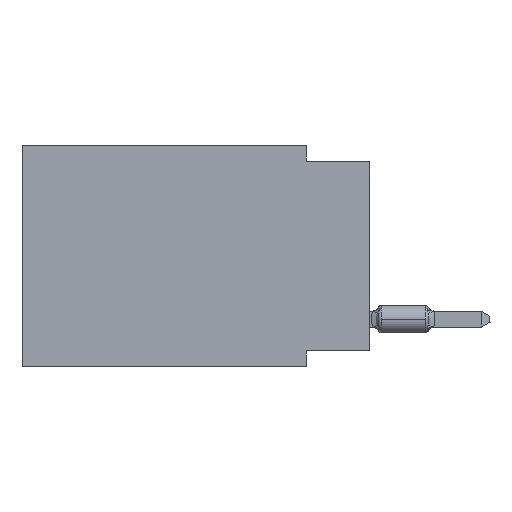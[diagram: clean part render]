
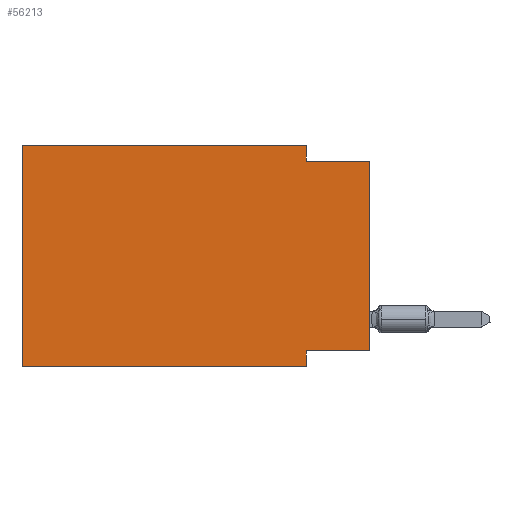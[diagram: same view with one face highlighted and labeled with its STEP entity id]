
A CAD part, left-side view. The second image highlights one B-rep face of the part: STEP entity #56213.
In plain terms, the highlighted planar face has unit normal (-1, 0, 0).
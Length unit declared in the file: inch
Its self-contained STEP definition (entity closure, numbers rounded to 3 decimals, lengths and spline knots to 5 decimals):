
#253 = VECTOR ( 'NONE', #26847, 39.37008 ) ;
#733 = VECTOR ( 'NONE', #78501, 39.37008 ) ;
#910 = LINE ( 'NONE', #87349, #33167 ) ;
#974 = VERTEX_POINT ( 'NONE', #85947 ) ;
#3097 = EDGE_LOOP ( 'NONE', ( #95310, #85120, #35525, #90242, #63247, #29142, #25572, #78518 ) ) ;
#9941 = DIRECTION ( 'NONE',  ( 0., 0., -1. ) ) ;
#10083 = CARTESIAN_POINT ( 'NONE',  ( 0., 0.1, 0. ) ) ;
#11758 = CARTESIAN_POINT ( 'NONE',  ( 0., 0.55, 0. ) ) ;
#11990 = EDGE_CURVE ( 'NONE', #82750, #92309, #94597, .T. ) ;
#13681 = VERTEX_POINT ( 'NONE', #62762 ) ;
#15347 = CARTESIAN_POINT ( 'NONE',  ( 0., 0.55, 0. ) ) ;
#17372 = DIRECTION ( 'NONE',  ( 0., 0., 1. ) ) ;
#17712 = EDGE_CURVE ( 'NONE', #47545, #46386, #76178, .T. ) ;
#20747 = DIRECTION ( 'NONE',  ( 0., -1., 0. ) ) ;
#23045 = EDGE_CURVE ( 'NONE', #47545, #87783, #51930, .T. ) ;
#25572 = ORIENTED_EDGE ( 'NONE', *, *, #84690, .F. ) ;
#26516 = CARTESIAN_POINT ( 'NONE',  ( 0., 0.55, -0.35 ) ) ;
#26847 = DIRECTION ( 'NONE',  ( 0., 1., 0. ) ) ;
#29142 = ORIENTED_EDGE ( 'NONE', *, *, #23045, .T. ) ;
#29228 = LINE ( 'NONE', #63686, #35225 ) ;
#31982 = VECTOR ( 'NONE', #103649, 39.37008 ) ;
#32868 = LINE ( 'NONE', #15347, #35991 ) ;
#33167 = VECTOR ( 'NONE', #9941, 39.37008 ) ;
#35225 = VECTOR ( 'NONE', #20747, 39.37008 ) ;
#35525 = ORIENTED_EDGE ( 'NONE', *, *, #102534, .F. ) ;
#35991 = VECTOR ( 'NONE', #67318, 39.37008 ) ;
#41147 = LINE ( 'NONE', #58653, #95939 ) ;
#46386 = VERTEX_POINT ( 'NONE', #98865 ) ;
#47545 = VERTEX_POINT ( 'NONE', #80386 ) ;
#50631 = LINE ( 'NONE', #85115, #253 ) ;
#51930 = LINE ( 'NONE', #26516, #733 ) ;
#54200 = VECTOR ( 'NONE', #17372, 39.37008 ) ;
#56213 = ADVANCED_FACE ( 'NONE', ( #89169 ), #103924, .F. ) ;
#58653 = CARTESIAN_POINT ( 'NONE',  ( 0., 0.1, 0. ) ) ;
#59770 = AXIS2_PLACEMENT_3D ( 'NONE', #11758, #69436, #60941 ) ;
#60941 = DIRECTION ( 'NONE',  ( 0., 0., -1. ) ) ;
#62762 = CARTESIAN_POINT ( 'NONE',  ( 0., 0.1, -0.025 ) ) ;
#63247 = ORIENTED_EDGE ( 'NONE', *, *, #17712, .F. ) ;
#63686 = CARTESIAN_POINT ( 'NONE',  ( 0., 0., -0.025 ) ) ;
#65373 = VERTEX_POINT ( 'NONE', #10083 ) ;
#67318 = DIRECTION ( 'NONE',  ( 0., -1., 0. ) ) ;
#69151 = CARTESIAN_POINT ( 'NONE',  ( 0., 0., 0. ) ) ;
#69436 = DIRECTION ( 'NONE',  ( 1., 0., 0. ) ) ;
#75622 = CARTESIAN_POINT ( 'NONE',  ( 0., 0.55, 0. ) ) ;
#76178 = LINE ( 'NONE', #75622, #54200 ) ;
#78501 = DIRECTION ( 'NONE',  ( 0., -1., 0. ) ) ;
#78518 = ORIENTED_EDGE ( 'NONE', *, *, #82233, .F. ) ;
#80386 = CARTESIAN_POINT ( 'NONE',  ( 0., 0.55, -0.35 ) ) ;
#82233 = EDGE_CURVE ( 'NONE', #82750, #974, #50631, .T. ) ;
#82750 = VERTEX_POINT ( 'NONE', #106791 ) ;
#83240 = CARTESIAN_POINT ( 'NONE',  ( 0., 0., -0.025 ) ) ;
#84690 = EDGE_CURVE ( 'NONE', #974, #87783, #910, .T. ) ;
#85115 = CARTESIAN_POINT ( 'NONE',  ( 0., 0., -0.325 ) ) ;
#85120 = ORIENTED_EDGE ( 'NONE', *, *, #87970, .F. ) ;
#85221 = DIRECTION ( 'NONE',  ( 0., 0., -1. ) ) ;
#85947 = CARTESIAN_POINT ( 'NONE',  ( 0., 0.1, -0.325 ) ) ;
#87349 = CARTESIAN_POINT ( 'NONE',  ( 0., 0.1, -0.35 ) ) ;
#87783 = VERTEX_POINT ( 'NONE', #111783 ) ;
#87970 = EDGE_CURVE ( 'NONE', #13681, #92309, #29228, .T. ) ;
#89169 = FACE_OUTER_BOUND ( 'NONE', #3097, .T. ) ;
#90242 = ORIENTED_EDGE ( 'NONE', *, *, #100379, .F. ) ;
#92309 = VERTEX_POINT ( 'NONE', #83240 ) ;
#94597 = LINE ( 'NONE', #69151, #31982 ) ;
#95310 = ORIENTED_EDGE ( 'NONE', *, *, #11990, .T. ) ;
#95939 = VECTOR ( 'NONE', #85221, 39.37008 ) ;
#98865 = CARTESIAN_POINT ( 'NONE',  ( 0., 0.55, 0. ) ) ;
#100379 = EDGE_CURVE ( 'NONE', #46386, #65373, #32868, .T. ) ;
#102534 = EDGE_CURVE ( 'NONE', #65373, #13681, #41147, .T. ) ;
#103649 = DIRECTION ( 'NONE',  ( 0., 0., 1. ) ) ;
#103924 = PLANE ( 'NONE',  #59770 ) ;
#106791 = CARTESIAN_POINT ( 'NONE',  ( 0., 0., -0.325 ) ) ;
#111783 = CARTESIAN_POINT ( 'NONE',  ( 0., 0.1, -0.35 ) ) ;
